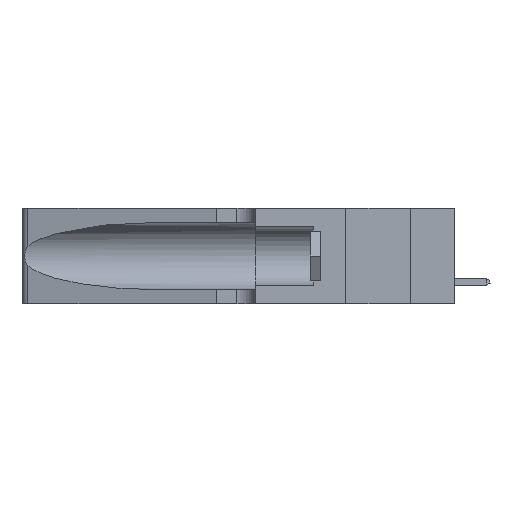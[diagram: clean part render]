
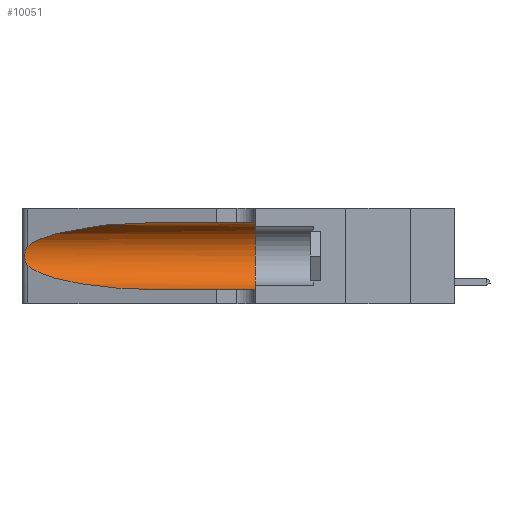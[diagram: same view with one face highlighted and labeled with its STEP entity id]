
A CAD part, left-side view. The second image highlights one B-rep face of the part: STEP entity #10051.
In plain terms, the highlighted cylindrical face has radius 3.308 mm (diameter 6.617 mm), a partial arc.
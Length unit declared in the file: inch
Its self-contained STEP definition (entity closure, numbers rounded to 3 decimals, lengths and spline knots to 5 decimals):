
#98 = CARTESIAN_POINT ( 'NONE',  ( 0.26017, 1.23833, 0.17102 ) ) ;
#176 = CARTESIAN_POINT ( 'NONE',  ( 0.26075, 1.23896, 0.19203 ) ) ;
#262 = DIRECTION ( 'NONE',  ( 0., 1., 0. ) ) ;
#2056 = CARTESIAN_POINT ( 'NONE',  ( 0.2373, 1.15595, 0.28018 ) ) ;
#2167 = CARTESIAN_POINT ( 'NONE',  ( 0.25487, 1.22718, 0.22369 ) ) ;
#3567 = EDGE_CURVE ( 'NONE', #18469, #10299, #12006, .T. ) ;
#4431 = CARTESIAN_POINT ( 'NONE',  ( 0.18966, 0.96281, 0.05475 ) ) ;
#4455 = CARTESIAN_POINT ( 'NONE',  ( 0.1305, 0.35, 0.31525 ) ) ;
#4464 = FACE_OUTER_BOUND ( 'NONE', #14351, .T. ) ;
#4613 = CARTESIAN_POINT ( 'NONE',  ( 0.1305, 0.72297, 0.05475 ) ) ;
#5260 = EDGE_CURVE ( 'NONE', #7154, #19501, #23829, .T. ) ;
#5262 = CARTESIAN_POINT ( 'NONE',  ( 0.1305, 1.61858, 0.185 ) ) ;
#5782 = DIRECTION ( 'NONE',  ( 0., 0., -1. ) ) ;
#5895 = VERTEX_POINT ( 'NONE', #13230 ) ;
#5903 = EDGE_CURVE ( 'NONE', #19501, #5895, #20215, .T. ) ;
#6329 = ORIENTED_EDGE ( 'NONE', *, *, #16948, .T. ) ;
#7154 = VERTEX_POINT ( 'NONE', #13321 ) ;
#7543 = CARTESIAN_POINT ( 'NONE',  ( 0.25856, 1.23593, 0.16098 ) ) ;
#8226 = LINE ( 'NONE', #10166, #10326 ) ;
#9404 = AXIS2_PLACEMENT_3D ( 'NONE', #15597, #262, #13477 ) ;
#9693 = CARTESIAN_POINT ( 'NONE',  ( 0.1305, 0.72297, 0.31525 ) ) ;
#9841 = CARTESIAN_POINT ( 'NONE',  ( 0.25487, 1.22718, 0.14631 ) ) ;
#10051 = ADVANCED_FACE ( 'NONE', ( #4464 ), #14047, .F. ) ;
#10166 = CARTESIAN_POINT ( 'NONE',  ( 0.1305, 1.61858, 0.05475 ) ) ;
#10299 = VERTEX_POINT ( 'NONE', #22277 ) ;
#10326 = VECTOR ( 'NONE', #21928, 39.37008 ) ;
#11152 = VECTOR ( 'NONE', #11262, 39.37008 ) ;
#11256 = VERTEX_POINT ( 'NONE', #23222 ) ;
#11262 = DIRECTION ( 'NONE',  ( 0., -1., 0. ) ) ;
#11285 = CARTESIAN_POINT ( 'NONE',  ( 0.25487, 1.22718, 0.22369 ) ) ;
#11528 = CARTESIAN_POINT ( 'NONE',  ( 0.25787, 1.23484, 0.2124 ) ) ;
#11704 = CARTESIAN_POINT ( 'NONE',  ( 0.25789, 1.23486, 0.15765 ) ) ;
#11717 = EDGE_CURVE ( 'NONE', #5895, #11256, #18231, .T. ) ;
#11989 = ORIENTED_EDGE ( 'NONE', *, *, #5903, .T. ) ;
#12006 = CIRCLE ( 'NONE', #9404, 0.13025 ) ;
#13230 = CARTESIAN_POINT ( 'NONE',  ( 0.25487, 1.22718, 0.14631 ) ) ;
#13321 = CARTESIAN_POINT ( 'NONE',  ( 0.1305, 0.72297, 0.31525 ) ) ;
#13475 = CARTESIAN_POINT ( 'NONE',  ( 0.25854, 1.2359, 0.20912 ) ) ;
#13477 = DIRECTION ( 'NONE',  ( 0., 0., 1. ) ) ;
#13561 = CARTESIAN_POINT ( 'NONE',  ( 0.25639, 1.23186, 0.15144 ) ) ;
#13612 = CARTESIAN_POINT ( 'NONE',  ( 0.2373, 1.15595, 0.08982 ) ) ;
#14047 = CYLINDRICAL_SURFACE ( 'NONE', #16002, 0.13025 ) ;
#14351 = EDGE_LOOP ( 'NONE', ( #23348, #11989, #18558, #6329, #14678, #19703 ) ) ;
#14678 = ORIENTED_EDGE ( 'NONE', *, *, #3567, .F. ) ;
#15417 = CARTESIAN_POINT ( 'NONE',  ( 0.25487, 1.22718, 0.14631 ) ) ;
#15597 = CARTESIAN_POINT ( 'NONE',  ( 0.1305, 0.35, 0.185 ) ) ;
#16002 = AXIS2_PLACEMENT_3D ( 'NONE', #5262, #16562, #5782 ) ;
#16562 = DIRECTION ( 'NONE',  ( 0., -1., 0. ) ) ;
#16620 = CARTESIAN_POINT ( 'NONE',  ( 0.1305, 1.61858, 0.31525 ) ) ;
#16948 = EDGE_CURVE ( 'NONE', #11256, #10299, #8226, .T. ) ;
#17206 = CARTESIAN_POINT ( 'NONE',  ( 0.26075, 1.23896, 0.178 ) ) ;
#17445 = CARTESIAN_POINT ( 'NONE',  ( 0.25555, 1.22993, 0.14849 ) ) ;
#18023 = EDGE_CURVE ( 'NONE', #7154, #18469, #19229, .T. ) ;
#18231 =( BOUNDED_CURVE ( )  B_SPLINE_CURVE ( 3, ( #9841, #13612, #4431, #4613 ),
 .UNSPECIFIED., .F., .T. ) 
 B_SPLINE_CURVE_WITH_KNOTS ( ( 4, 4 ),
 ( 3.44316, 4.71239 ),
 .UNSPECIFIED. ) 
 CURVE ( )  GEOMETRIC_REPRESENTATION_ITEM ( )  RATIONAL_B_SPLINE_CURVE ( ( 1., 0.87, 0.87, 1. ) ) 
 REPRESENTATION_ITEM ( '' )  );
#18469 = VERTEX_POINT ( 'NONE', #4455 ) ;
#18558 = ORIENTED_EDGE ( 'NONE', *, *, #11717, .T. ) ;
#19005 = CARTESIAN_POINT ( 'NONE',  ( 0.18966, 0.96281, 0.31525 ) ) ;
#19229 = LINE ( 'NONE', #16620, #11152 ) ;
#19325 = CARTESIAN_POINT ( 'NONE',  ( 0.25639, 1.23184, 0.21858 ) ) ;
#19501 = VERTEX_POINT ( 'NONE', #23376 ) ;
#19703 = ORIENTED_EDGE ( 'NONE', *, *, #18023, .F. ) ;
#20215 = B_SPLINE_CURVE_WITH_KNOTS ( 'NONE', 3,
 ( #2167, #21081, #19325, #11528, #13475, #22971, #176, #17206, #98, #7543, #11704, #13561, #17445, #15417 ),
 .UNSPECIFIED., .F., .F.,
 ( 4, 2, 2, 2, 2, 2, 4 ),
 ( 0., 0.00027, 0.00053, 0.00107, 0.0016, 0.00187, 0.00214 ),
 .UNSPECIFIED. ) ;
#21081 = CARTESIAN_POINT ( 'NONE',  ( 0.25555, 1.22994, 0.2215 ) ) ;
#21928 = DIRECTION ( 'NONE',  ( 0., -1., 0. ) ) ;
#22277 = CARTESIAN_POINT ( 'NONE',  ( 0.1305, 0.35, 0.05475 ) ) ;
#22971 = CARTESIAN_POINT ( 'NONE',  ( 0.26018, 1.23835, 0.19895 ) ) ;
#23222 = CARTESIAN_POINT ( 'NONE',  ( 0.1305, 0.72297, 0.05475 ) ) ;
#23348 = ORIENTED_EDGE ( 'NONE', *, *, #5260, .T. ) ;
#23376 = CARTESIAN_POINT ( 'NONE',  ( 0.25487, 1.22718, 0.22369 ) ) ;
#23829 =( BOUNDED_CURVE ( )  B_SPLINE_CURVE ( 3, ( #9693, #19005, #2056, #11285 ),
 .UNSPECIFIED., .F., .T. ) 
 B_SPLINE_CURVE_WITH_KNOTS ( ( 4, 4 ),
 ( 1.5708, 2.84003 ),
 .UNSPECIFIED. ) 
 CURVE ( )  GEOMETRIC_REPRESENTATION_ITEM ( )  RATIONAL_B_SPLINE_CURVE ( ( 1., 0.87, 0.87, 1. ) ) 
 REPRESENTATION_ITEM ( '' )  );
